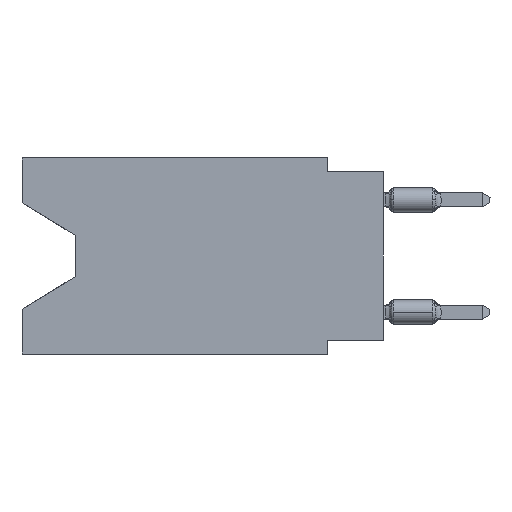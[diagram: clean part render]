
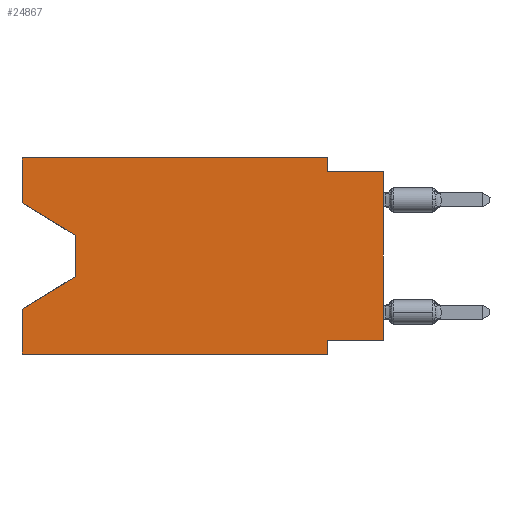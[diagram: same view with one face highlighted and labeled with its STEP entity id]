
A CAD part, left-side view. The second image highlights one B-rep face of the part: STEP entity #24867.
In plain terms, the highlighted planar face has unit normal (-1, 0, 0).
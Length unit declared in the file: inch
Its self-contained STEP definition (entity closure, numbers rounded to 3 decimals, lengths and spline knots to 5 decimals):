
#915 = CARTESIAN_POINT ( 'NONE',  ( 0., 0.1, 0. ) ) ;
#1740 = CARTESIAN_POINT ( 'NONE',  ( 0., 0., -0.325 ) ) ;
#3217 = ORIENTED_EDGE ( 'NONE', *, *, #16349, .F. ) ;
#3282 = EDGE_CURVE ( 'NONE', #16975, #22232, #31629, .T. ) ;
#3433 = CARTESIAN_POINT ( 'NONE',  ( 0., 0., -0.325 ) ) ;
#3599 = CARTESIAN_POINT ( 'NONE',  ( 0., 0.645, -0.08025 ) ) ;
#3615 = CARTESIAN_POINT ( 'NONE',  ( 0., 0., 0. ) ) ;
#3775 = VERTEX_POINT ( 'NONE', #27461 ) ;
#4671 = CARTESIAN_POINT ( 'NONE',  ( 0., 0., -0.025 ) ) ;
#4767 = EDGE_CURVE ( 'NONE', #18400, #3775, #25202, .T. ) ;
#4906 = ORIENTED_EDGE ( 'NONE', *, *, #25542, .F. ) ;
#5194 = CARTESIAN_POINT ( 'NONE',  ( 0., 0.645, 0. ) ) ;
#5318 = LINE ( 'NONE', #1740, #21187 ) ;
#5395 = CARTESIAN_POINT ( 'NONE',  ( 0., 0.645, 0. ) ) ;
#6059 = LINE ( 'NONE', #3599, #30835 ) ;
#6197 = CARTESIAN_POINT ( 'NONE',  ( 0., 0., -0.025 ) ) ;
#6598 = CARTESIAN_POINT ( 'NONE',  ( 0., 0.55, -0.212 ) ) ;
#6688 = CARTESIAN_POINT ( 'NONE',  ( 0., 0.645, -0.26975 ) ) ;
#7136 = LINE ( 'NONE', #4671, #8482 ) ;
#7676 = VECTOR ( 'NONE', #30286, 39.37008 ) ;
#7803 = LINE ( 'NONE', #10738, #18024 ) ;
#7861 = VECTOR ( 'NONE', #13143, 39.37008 ) ;
#7913 = CARTESIAN_POINT ( 'NONE',  ( 0., 0.645, 0. ) ) ;
#8482 = VECTOR ( 'NONE', #17705, 39.37008 ) ;
#9628 = LINE ( 'NONE', #32398, #18278 ) ;
#10738 = CARTESIAN_POINT ( 'NONE',  ( 0., 0.645, 0. ) ) ;
#11186 = VECTOR ( 'NONE', #18936, 39.37008 ) ;
#11484 = VERTEX_POINT ( 'NONE', #3433 ) ;
#11796 = DIRECTION ( 'NONE',  ( 0., 1., 0. ) ) ;
#12629 = DIRECTION ( 'NONE',  ( 0., 0., -1. ) ) ;
#12669 = CARTESIAN_POINT ( 'NONE',  ( 0., 0.55, -0.138 ) ) ;
#12779 = PLANE ( 'NONE',  #21026 ) ;
#12808 = CARTESIAN_POINT ( 'NONE',  ( 0., 0.645, -0.35 ) ) ;
#13143 = DIRECTION ( 'NONE',  ( 0., 0., -1. ) ) ;
#13284 = ORIENTED_EDGE ( 'NONE', *, *, #18647, .T. ) ;
#13656 = VECTOR ( 'NONE', #17611, 39.37008 ) ;
#13732 = ORIENTED_EDGE ( 'NONE', *, *, #3282, .T. ) ;
#14720 = VERTEX_POINT ( 'NONE', #6197 ) ;
#14777 = DIRECTION ( 'NONE',  ( 1., 0., 0. ) ) ;
#14934 = FACE_OUTER_BOUND ( 'NONE', #15090, .T. ) ;
#15090 = EDGE_LOOP ( 'NONE', ( #13284, #13732, #28191, #21060, #30590, #31440, #15933, #23727, #25878, #4906, #3217, #23543 ) ) ;
#15873 = CARTESIAN_POINT ( 'NONE',  ( 0., 0.645, -0.08025 ) ) ;
#15933 = ORIENTED_EDGE ( 'NONE', *, *, #28363, .F. ) ;
#16303 = DIRECTION ( 'NONE',  ( 0., -0.855, -0.519 ) ) ;
#16349 = EDGE_CURVE ( 'NONE', #28161, #29014, #9628, .T. ) ;
#16975 = VERTEX_POINT ( 'NONE', #12669 ) ;
#17351 = CARTESIAN_POINT ( 'NONE',  ( 0., 0.1, -0.025 ) ) ;
#17611 = DIRECTION ( 'NONE',  ( 0., -1., 0. ) ) ;
#17705 = DIRECTION ( 'NONE',  ( 0., -1., 0. ) ) ;
#17974 = DIRECTION ( 'NONE',  ( 0., 0., 1. ) ) ;
#18024 = VECTOR ( 'NONE', #30712, 39.37008 ) ;
#18278 = VECTOR ( 'NONE', #29417, 39.37008 ) ;
#18400 = VERTEX_POINT ( 'NONE', #31108 ) ;
#18647 = EDGE_CURVE ( 'NONE', #26783, #16975, #6059, .T. ) ;
#18936 = DIRECTION ( 'NONE',  ( 0., 0., -1. ) ) ;
#19083 = VECTOR ( 'NONE', #21269, 39.37008 ) ;
#20232 = CARTESIAN_POINT ( 'NONE',  ( 0., 0.1, -0.35 ) ) ;
#20286 = EDGE_CURVE ( 'NONE', #26601, #30137, #30502, .T. ) ;
#20341 = CARTESIAN_POINT ( 'NONE',  ( 0., 0.1, 0. ) ) ;
#21026 = AXIS2_PLACEMENT_3D ( 'NONE', #5194, #14777, #12629 ) ;
#21060 = ORIENTED_EDGE ( 'NONE', *, *, #20286, .F. ) ;
#21187 = VECTOR ( 'NONE', #11796, 39.37008 ) ;
#21269 = DIRECTION ( 'NONE',  ( 0., 0., 1. ) ) ;
#21644 = LINE ( 'NONE', #6598, #31556 ) ;
#22232 = VERTEX_POINT ( 'NONE', #30659 ) ;
#22439 = LINE ( 'NONE', #915, #7861 ) ;
#22560 = VECTOR ( 'NONE', #17974, 39.37008 ) ;
#22701 = EDGE_CURVE ( 'NONE', #26601, #3775, #28293, .T. ) ;
#23523 = EDGE_CURVE ( 'NONE', #22232, #30137, #21644, .T. ) ;
#23543 = ORIENTED_EDGE ( 'NONE', *, *, #30934, .F. ) ;
#23604 = VERTEX_POINT ( 'NONE', #17351 ) ;
#23727 = ORIENTED_EDGE ( 'NONE', *, *, #30821, .T. ) ;
#23906 = LINE ( 'NONE', #3615, #19083 ) ;
#24259 = CARTESIAN_POINT ( 'NONE',  ( 0., 0.645, -0.35 ) ) ;
#24867 = ADVANCED_FACE ( 'NONE', ( #14934 ), #12779, .F. ) ;
#25202 = LINE ( 'NONE', #20232, #7676 ) ;
#25542 = EDGE_CURVE ( 'NONE', #29014, #23604, #22439, .T. ) ;
#25878 = ORIENTED_EDGE ( 'NONE', *, *, #28976, .F. ) ;
#26601 = VERTEX_POINT ( 'NONE', #24259 ) ;
#26783 = VERTEX_POINT ( 'NONE', #15873 ) ;
#27461 = CARTESIAN_POINT ( 'NONE',  ( 0., 0.1, -0.35 ) ) ;
#28161 = VERTEX_POINT ( 'NONE', #5395 ) ;
#28191 = ORIENTED_EDGE ( 'NONE', *, *, #23523, .T. ) ;
#28293 = LINE ( 'NONE', #12808, #13656 ) ;
#28363 = EDGE_CURVE ( 'NONE', #11484, #18400, #5318, .T. ) ;
#28976 = EDGE_CURVE ( 'NONE', #23604, #14720, #7136, .T. ) ;
#29014 = VERTEX_POINT ( 'NONE', #20341 ) ;
#29417 = DIRECTION ( 'NONE',  ( 0., -1., 0. ) ) ;
#30137 = VERTEX_POINT ( 'NONE', #6688 ) ;
#30286 = DIRECTION ( 'NONE',  ( 0., 0., -1. ) ) ;
#30502 = LINE ( 'NONE', #7913, #22560 ) ;
#30590 = ORIENTED_EDGE ( 'NONE', *, *, #22701, .T. ) ;
#30659 = CARTESIAN_POINT ( 'NONE',  ( 0., 0.55, -0.212 ) ) ;
#30712 = DIRECTION ( 'NONE',  ( 0., 0., 1. ) ) ;
#30821 = EDGE_CURVE ( 'NONE', #11484, #14720, #23906, .T. ) ;
#30835 = VECTOR ( 'NONE', #16303, 39.37008 ) ;
#30934 = EDGE_CURVE ( 'NONE', #26783, #28161, #7803, .T. ) ;
#31108 = CARTESIAN_POINT ( 'NONE',  ( 0., 0.1, -0.325 ) ) ;
#31440 = ORIENTED_EDGE ( 'NONE', *, *, #4767, .F. ) ;
#31457 = CARTESIAN_POINT ( 'NONE',  ( 0., 0.55, -0.138 ) ) ;
#31556 = VECTOR ( 'NONE', #31691, 39.37008 ) ;
#31629 = LINE ( 'NONE', #31457, #11186 ) ;
#31691 = DIRECTION ( 'NONE',  ( 0., 0.855, -0.519 ) ) ;
#32398 = CARTESIAN_POINT ( 'NONE',  ( 0., 0.645, 0. ) ) ;
